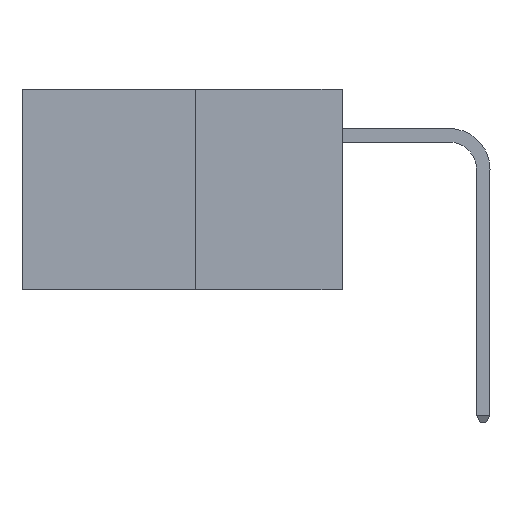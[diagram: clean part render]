
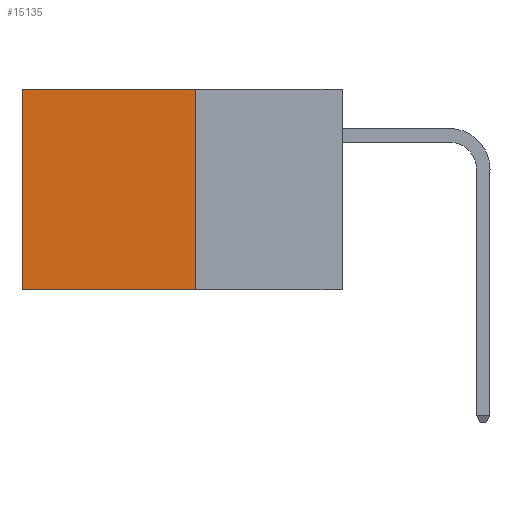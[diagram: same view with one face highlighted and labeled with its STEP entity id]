
A CAD part, left-side view. The second image highlights one B-rep face of the part: STEP entity #15135.
In plain terms, the highlighted planar face has unit normal (-1, 0, 0).
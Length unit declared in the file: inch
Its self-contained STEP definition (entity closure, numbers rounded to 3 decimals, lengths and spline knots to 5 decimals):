
#537 = PLANE ( 'NONE',  #13723 ) ;
#590 = CARTESIAN_POINT ( 'NONE',  ( 0.277, 0.59, -0.37 ) ) ;
#1074 = LINE ( 'NONE', #12291, #11348 ) ;
#2094 = DIRECTION ( 'NONE',  ( 0., 0., -1. ) ) ;
#3653 = EDGE_LOOP ( 'NONE', ( #16909, #16925, #15962, #15386 ) ) ;
#3776 = CARTESIAN_POINT ( 'NONE',  ( 0.277, 0.27, -0.37 ) ) ;
#3859 = VERTEX_POINT ( 'NONE', #7892 ) ;
#4583 = DIRECTION ( 'NONE',  ( 1., 0., 0. ) ) ;
#5934 = LINE ( 'NONE', #14796, #12475 ) ;
#6621 = CARTESIAN_POINT ( 'NONE',  ( 0.277, 0.27, 0. ) ) ;
#6782 = VERTEX_POINT ( 'NONE', #590 ) ;
#7498 = LINE ( 'NONE', #3776, #10564 ) ;
#7668 = FACE_OUTER_BOUND ( 'NONE', #3653, .T. ) ;
#7676 = LINE ( 'NONE', #13264, #9900 ) ;
#7879 = DIRECTION ( 'NONE',  ( 0., 0., -1. ) ) ;
#7892 = CARTESIAN_POINT ( 'NONE',  ( 0.277, 0.27, -0.37 ) ) ;
#8989 = EDGE_CURVE ( 'NONE', #11403, #6782, #7676, .T. ) ;
#9900 = VECTOR ( 'NONE', #2094, 39.37008 ) ;
#9990 = DIRECTION ( 'NONE',  ( 0., 0., -1. ) ) ;
#10298 = EDGE_CURVE ( 'NONE', #14296, #11403, #5934, .T. ) ;
#10564 = VECTOR ( 'NONE', #7879, 39.37008 ) ;
#11348 = VECTOR ( 'NONE', #16021, 39.37008 ) ;
#11403 = VERTEX_POINT ( 'NONE', #15128 ) ;
#12291 = CARTESIAN_POINT ( 'NONE',  ( 0.277, 0.27, -0.37 ) ) ;
#12475 = VECTOR ( 'NONE', #14905, 39.37008 ) ;
#13264 = CARTESIAN_POINT ( 'NONE',  ( 0.277, 0.59, -0.37 ) ) ;
#13723 = AXIS2_PLACEMENT_3D ( 'NONE', #16219, #4583, #9990 ) ;
#14296 = VERTEX_POINT ( 'NONE', #6621 ) ;
#14544 = EDGE_CURVE ( 'NONE', #3859, #6782, #1074, .T. ) ;
#14796 = CARTESIAN_POINT ( 'NONE',  ( 0.277, 0.27, 0. ) ) ;
#14905 = DIRECTION ( 'NONE',  ( 0., 1., 0. ) ) ;
#15128 = CARTESIAN_POINT ( 'NONE',  ( 0.277, 0.59, 0. ) ) ;
#15135 = ADVANCED_FACE ( 'NONE', ( #7668 ), #537, .F. ) ;
#15386 = ORIENTED_EDGE ( 'NONE', *, *, #10298, .T. ) ;
#15962 = ORIENTED_EDGE ( 'NONE', *, *, #16532, .F. ) ;
#16021 = DIRECTION ( 'NONE',  ( 0., 1., 0. ) ) ;
#16219 = CARTESIAN_POINT ( 'NONE',  ( 0.277, 0.27, -0.37 ) ) ;
#16532 = EDGE_CURVE ( 'NONE', #14296, #3859, #7498, .T. ) ;
#16909 = ORIENTED_EDGE ( 'NONE', *, *, #8989, .T. ) ;
#16925 = ORIENTED_EDGE ( 'NONE', *, *, #14544, .F. ) ;
